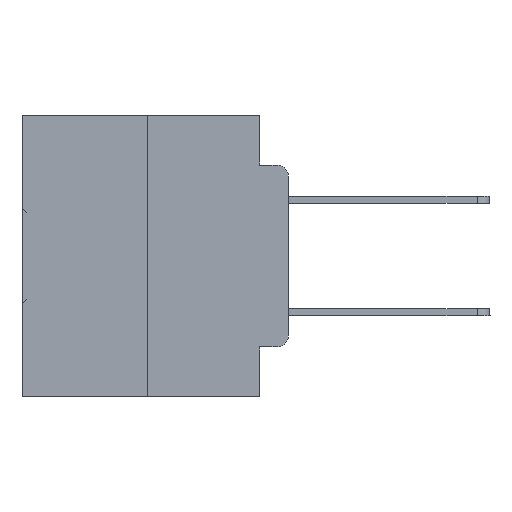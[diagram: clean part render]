
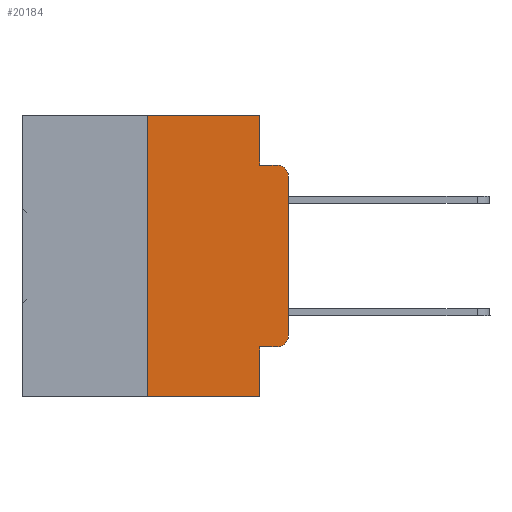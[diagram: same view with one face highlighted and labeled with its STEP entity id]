
A CAD part, left-side view. The second image highlights one B-rep face of the part: STEP entity #20184.
In plain terms, the highlighted planar face has unit normal (-1, 0, 0).
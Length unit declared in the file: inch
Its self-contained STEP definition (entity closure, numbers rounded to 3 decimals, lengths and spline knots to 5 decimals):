
#1252 = EDGE_LOOP ( 'NONE', ( #28984, #21590, #26662, #23892, #36346, #30080, #23369, #17744, #5349, #5119 ) ) ;
#1818 = LINE ( 'NONE', #15996, #27327 ) ;
#2041 = DIRECTION ( 'NONE',  ( 0., 0., 1. ) ) ;
#2057 = EDGE_CURVE ( 'NONE', #17048, #21482, #4106, .T. ) ;
#3572 = CARTESIAN_POINT ( 'NONE',  ( 0., 0.02, -0.0885 ) ) ;
#4102 = EDGE_CURVE ( 'NONE', #13290, #18979, #18330, .T. ) ;
#4106 = LINE ( 'NONE', #21684, #5052 ) ;
#4453 = DIRECTION ( 'NONE',  ( 0., 0., -1. ) ) ;
#4846 = CARTESIAN_POINT ( 'NONE',  ( 0., 0.051, -0.4115 ) ) ;
#5018 = DIRECTION ( 'NONE',  ( 0., 0., -1. ) ) ;
#5052 = VECTOR ( 'NONE', #16199, 39.37008 ) ;
#5119 = ORIENTED_EDGE ( 'NONE', *, *, #22722, .T. ) ;
#5120 = CARTESIAN_POINT ( 'NONE',  ( 0., 0.473, 0. ) ) ;
#5249 = PLANE ( 'NONE',  #26487 ) ;
#5349 = ORIENTED_EDGE ( 'NONE', *, *, #16396, .T. ) ;
#5370 = DIRECTION ( 'NONE',  ( 0., 0., -1. ) ) ;
#5587 = VECTOR ( 'NONE', #33371, 39.37008 ) ;
#6002 = LINE ( 'NONE', #33432, #35483 ) ;
#7557 = CARTESIAN_POINT ( 'NONE',  ( 0., 0., -0.3915 ) ) ;
#7720 = LINE ( 'NONE', #10824, #27413 ) ;
#7853 = VECTOR ( 'NONE', #21882, 39.37008 ) ;
#8046 = CARTESIAN_POINT ( 'NONE',  ( 0., 0., 0. ) ) ;
#8443 = VERTEX_POINT ( 'NONE', #10459 ) ;
#8617 = DIRECTION ( 'NONE',  ( 0., 0., -1. ) ) ;
#9040 = CARTESIAN_POINT ( 'NONE',  ( 0., 0.051, -0.0885 ) ) ;
#9775 = EDGE_CURVE ( 'NONE', #21027, #18979, #29277, .T. ) ;
#10071 = LINE ( 'NONE', #21637, #7853 ) ;
#10459 = CARTESIAN_POINT ( 'NONE',  ( 0., 0.02, -0.4115 ) ) ;
#10823 = EDGE_CURVE ( 'NONE', #30846, #13290, #31082, .T. ) ;
#10824 = CARTESIAN_POINT ( 'NONE',  ( 0., 0.051, 0. ) ) ;
#13290 = VERTEX_POINT ( 'NONE', #28055 ) ;
#13350 = EDGE_CURVE ( 'NONE', #21480, #17893, #6002, .T. ) ;
#13522 = AXIS2_PLACEMENT_3D ( 'NONE', #14032, #34304, #19868 ) ;
#14032 = CARTESIAN_POINT ( 'NONE',  ( 0., 0.02, -0.1085 ) ) ;
#14879 = LINE ( 'NONE', #21564, #5587 ) ;
#15996 = CARTESIAN_POINT ( 'NONE',  ( 0., 0.051, 0. ) ) ;
#16199 = DIRECTION ( 'NONE',  ( 0., -1., 0. ) ) ;
#16373 = DIRECTION ( 'NONE',  ( 0., -1., 0. ) ) ;
#16396 = EDGE_CURVE ( 'NONE', #27149, #8443, #14879, .T. ) ;
#17048 = VERTEX_POINT ( 'NONE', #24991 ) ;
#17079 = CARTESIAN_POINT ( 'NONE',  ( 0., 0.051, -0.5 ) ) ;
#17628 = VECTOR ( 'NONE', #25355, 39.37008 ) ;
#17644 = AXIS2_PLACEMENT_3D ( 'NONE', #19944, #25706, #8617 ) ;
#17744 = ORIENTED_EDGE ( 'NONE', *, *, #23617, .F. ) ;
#17893 = VERTEX_POINT ( 'NONE', #17079 ) ;
#18330 = CIRCLE ( 'NONE', #13522, 0.02 ) ;
#18979 = VERTEX_POINT ( 'NONE', #3572 ) ;
#19868 = DIRECTION ( 'NONE',  ( 0., 0., -1. ) ) ;
#19944 = CARTESIAN_POINT ( 'NONE',  ( 0., 0.02, -0.3915 ) ) ;
#20184 = ADVANCED_FACE ( 'NONE', ( #36103 ), #5249, .F. ) ;
#20654 = CARTESIAN_POINT ( 'NONE',  ( 0., 0.25, -0.5 ) ) ;
#21027 = VERTEX_POINT ( 'NONE', #9040 ) ;
#21188 = EDGE_CURVE ( 'NONE', #21480, #17048, #10071, .T. ) ;
#21480 = VERTEX_POINT ( 'NONE', #20654 ) ;
#21482 = VERTEX_POINT ( 'NONE', #29456 ) ;
#21564 = CARTESIAN_POINT ( 'NONE',  ( 0., 0.051, -0.4115 ) ) ;
#21590 = ORIENTED_EDGE ( 'NONE', *, *, #4102, .T. ) ;
#21637 = CARTESIAN_POINT ( 'NONE',  ( 0., 0.25, 0. ) ) ;
#21684 = CARTESIAN_POINT ( 'NONE',  ( 0., 0.473, 0. ) ) ;
#21882 = DIRECTION ( 'NONE',  ( 0., 0., 1. ) ) ;
#21999 = CIRCLE ( 'NONE', #17644, 0.02 ) ;
#22722 = EDGE_CURVE ( 'NONE', #8443, #30846, #21999, .T. ) ;
#23369 = ORIENTED_EDGE ( 'NONE', *, *, #13350, .T. ) ;
#23377 = VECTOR ( 'NONE', #2041, 39.37008 ) ;
#23617 = EDGE_CURVE ( 'NONE', #27149, #17893, #1818, .T. ) ;
#23892 = ORIENTED_EDGE ( 'NONE', *, *, #33962, .F. ) ;
#24991 = CARTESIAN_POINT ( 'NONE',  ( 0., 0.25, 0. ) ) ;
#25044 = DIRECTION ( 'NONE',  ( 1., 0., 0. ) ) ;
#25355 = DIRECTION ( 'NONE',  ( 0., -1., 0. ) ) ;
#25706 = DIRECTION ( 'NONE',  ( -1., 0., 0. ) ) ;
#26487 = AXIS2_PLACEMENT_3D ( 'NONE', #5120, #25044, #5370 ) ;
#26662 = ORIENTED_EDGE ( 'NONE', *, *, #9775, .F. ) ;
#27149 = VERTEX_POINT ( 'NONE', #4846 ) ;
#27327 = VECTOR ( 'NONE', #4453, 39.37008 ) ;
#27413 = VECTOR ( 'NONE', #5018, 39.37008 ) ;
#28055 = CARTESIAN_POINT ( 'NONE',  ( 0., 0., -0.1085 ) ) ;
#28984 = ORIENTED_EDGE ( 'NONE', *, *, #10823, .T. ) ;
#29277 = LINE ( 'NONE', #30989, #17628 ) ;
#29456 = CARTESIAN_POINT ( 'NONE',  ( 0., 0.051, 0. ) ) ;
#30080 = ORIENTED_EDGE ( 'NONE', *, *, #21188, .F. ) ;
#30846 = VERTEX_POINT ( 'NONE', #7557 ) ;
#30989 = CARTESIAN_POINT ( 'NONE',  ( 0., 0.051, -0.0885 ) ) ;
#31082 = LINE ( 'NONE', #8046, #23377 ) ;
#33371 = DIRECTION ( 'NONE',  ( 0., -1., 0. ) ) ;
#33432 = CARTESIAN_POINT ( 'NONE',  ( 0., 0.473, -0.5 ) ) ;
#33962 = EDGE_CURVE ( 'NONE', #21482, #21027, #7720, .T. ) ;
#34304 = DIRECTION ( 'NONE',  ( -1., 0., 0. ) ) ;
#35483 = VECTOR ( 'NONE', #16373, 39.37008 ) ;
#36103 = FACE_OUTER_BOUND ( 'NONE', #1252, .T. ) ;
#36346 = ORIENTED_EDGE ( 'NONE', *, *, #2057, .F. ) ;
